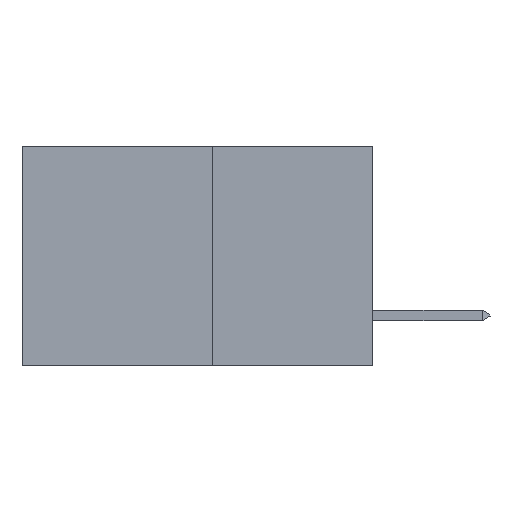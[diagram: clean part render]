
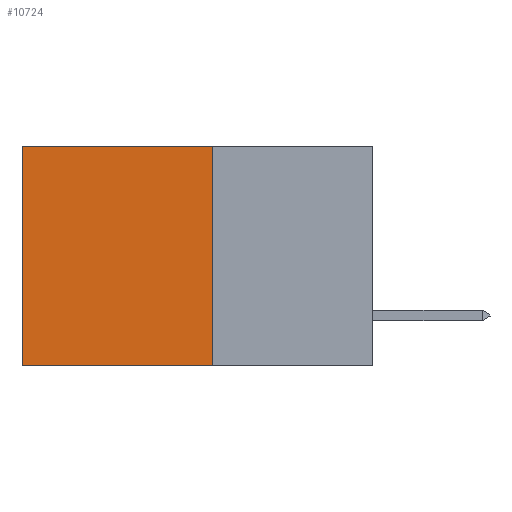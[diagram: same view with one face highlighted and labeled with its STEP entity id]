
A CAD part, left-side view. The second image highlights one B-rep face of the part: STEP entity #10724.
In plain terms, the highlighted planar face has unit normal (-1, 0, 0).
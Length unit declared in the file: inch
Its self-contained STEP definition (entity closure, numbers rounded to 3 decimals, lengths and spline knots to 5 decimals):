
#306 = VECTOR ( 'NONE', #15201, 39.37008 ) ;
#432 = VERTEX_POINT ( 'NONE', #8494 ) ;
#555 = CARTESIAN_POINT ( 'NONE',  ( 0.277, 0.27, -0.37 ) ) ;
#1719 = LINE ( 'NONE', #7288, #8007 ) ;
#1898 = ORIENTED_EDGE ( 'NONE', *, *, #2700, .T. ) ;
#2700 = EDGE_CURVE ( 'NONE', #4492, #5497, #11495, .T. ) ;
#3086 = LINE ( 'NONE', #555, #9459 ) ;
#3257 = DIRECTION ( 'NONE',  ( 0., 1., 0. ) ) ;
#3720 = DIRECTION ( 'NONE',  ( 1., 0., 0. ) ) ;
#4492 = VERTEX_POINT ( 'NONE', #7300 ) ;
#4729 = EDGE_LOOP ( 'NONE', ( #7780, #11142, #14419, #1898 ) ) ;
#5497 = VERTEX_POINT ( 'NONE', #10554 ) ;
#6019 = FACE_OUTER_BOUND ( 'NONE', #4729, .T. ) ;
#7288 = CARTESIAN_POINT ( 'NONE',  ( 0.277, 0.59, -0.37 ) ) ;
#7300 = CARTESIAN_POINT ( 'NONE',  ( 0.277, 0.27, 0. ) ) ;
#7503 = CARTESIAN_POINT ( 'NONE',  ( 0.277, 0.27, 0. ) ) ;
#7758 = CARTESIAN_POINT ( 'NONE',  ( 0.277, 0.27, -0.37 ) ) ;
#7773 = VECTOR ( 'NONE', #3257, 39.37008 ) ;
#7780 = ORIENTED_EDGE ( 'NONE', *, *, #11854, .T. ) ;
#8007 = VECTOR ( 'NONE', #9883, 39.37008 ) ;
#8494 = CARTESIAN_POINT ( 'NONE',  ( 0.277, 0.27, -0.37 ) ) ;
#8701 = AXIS2_PLACEMENT_3D ( 'NONE', #14930, #3720, #12489 ) ;
#9387 = CARTESIAN_POINT ( 'NONE',  ( 0.277, 0.59, -0.37 ) ) ;
#9459 = VECTOR ( 'NONE', #10613, 39.37008 ) ;
#9883 = DIRECTION ( 'NONE',  ( 0., 0., -1. ) ) ;
#10554 = CARTESIAN_POINT ( 'NONE',  ( 0.277, 0.59, 0. ) ) ;
#10613 = DIRECTION ( 'NONE',  ( 0., 1., 0. ) ) ;
#10724 = ADVANCED_FACE ( 'NONE', ( #6019 ), #16138, .F. ) ;
#11142 = ORIENTED_EDGE ( 'NONE', *, *, #11525, .F. ) ;
#11495 = LINE ( 'NONE', #7503, #7773 ) ;
#11525 = EDGE_CURVE ( 'NONE', #432, #13802, #3086, .T. ) ;
#11854 = EDGE_CURVE ( 'NONE', #5497, #13802, #1719, .T. ) ;
#12489 = DIRECTION ( 'NONE',  ( 0., 0., -1. ) ) ;
#13616 = LINE ( 'NONE', #7758, #306 ) ;
#13802 = VERTEX_POINT ( 'NONE', #9387 ) ;
#14419 = ORIENTED_EDGE ( 'NONE', *, *, #15085, .F. ) ;
#14930 = CARTESIAN_POINT ( 'NONE',  ( 0.277, 0.27, -0.37 ) ) ;
#15085 = EDGE_CURVE ( 'NONE', #4492, #432, #13616, .T. ) ;
#15201 = DIRECTION ( 'NONE',  ( 0., 0., -1. ) ) ;
#16138 = PLANE ( 'NONE',  #8701 ) ;
